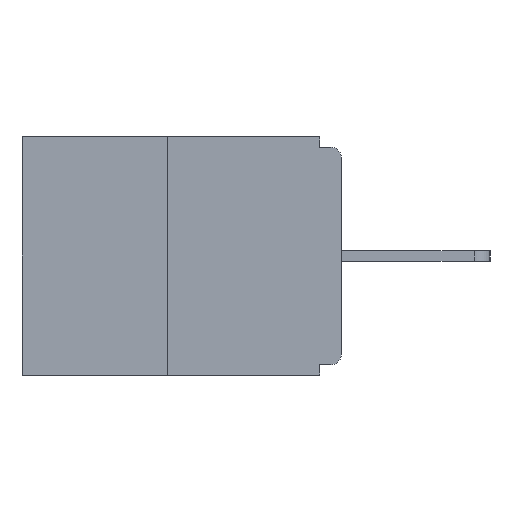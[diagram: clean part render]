
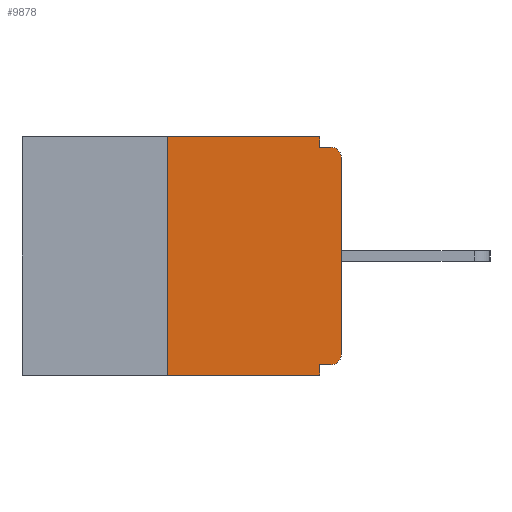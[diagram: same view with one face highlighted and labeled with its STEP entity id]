
A CAD part, left-side view. The second image highlights one B-rep face of the part: STEP entity #9878.
In plain terms, the highlighted planar face has unit normal (-1, 0, 0).
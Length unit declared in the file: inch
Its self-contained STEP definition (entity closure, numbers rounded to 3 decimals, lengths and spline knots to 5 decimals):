
#17 = CARTESIAN_POINT ( 'NONE',  ( 0., 0.25, 0. ) ) ;
#235 = DIRECTION ( 'NONE',  ( 0., 0., -1. ) ) ;
#285 = ORIENTED_EDGE ( 'NONE', *, *, #393, .F. ) ;
#359 = CARTESIAN_POINT ( 'NONE',  ( 0., 0.46, 0. ) ) ;
#393 = EDGE_CURVE ( 'NONE', #5378, #787, #4287, .T. ) ;
#433 = CARTESIAN_POINT ( 'NONE',  ( 0., 0.031, 0. ) ) ;
#787 = VERTEX_POINT ( 'NONE', #4577 ) ;
#872 = DIRECTION ( 'NONE',  ( 0., 0., -1. ) ) ;
#950 = LINE ( 'NONE', #11605, #6314 ) ;
#1039 = CARTESIAN_POINT ( 'NONE',  ( 0., 0.031, -0.015 ) ) ;
#1053 = PLANE ( 'NONE',  #10381 ) ;
#1226 = CARTESIAN_POINT ( 'NONE',  ( 0., 0.031, -0.343 ) ) ;
#1510 = VECTOR ( 'NONE', #7937, 39.37008 ) ;
#1736 = VERTEX_POINT ( 'NONE', #4170 ) ;
#2006 = VERTEX_POINT ( 'NONE', #6534 ) ;
#2143 = DIRECTION ( 'NONE',  ( 0., 0., 1. ) ) ;
#2172 = VERTEX_POINT ( 'NONE', #17 ) ;
#2188 = CARTESIAN_POINT ( 'NONE',  ( 0., 0., -0.015 ) ) ;
#2247 = VECTOR ( 'NONE', #2143, 39.37008 ) ;
#2302 = CARTESIAN_POINT ( 'NONE',  ( 0., 0.015, -0.03 ) ) ;
#2700 = AXIS2_PLACEMENT_3D ( 'NONE', #12912, #8951, #4931 ) ;
#2764 = EDGE_LOOP ( 'NONE', ( #7004, #6138, #12040, #3633, #285, #4777, #11546, #6437, #5167, #11574 ) ) ;
#2909 = CARTESIAN_POINT ( 'NONE',  ( 0., 0., 0. ) ) ;
#3272 = VECTOR ( 'NONE', #4357, 39.37008 ) ;
#3365 = EDGE_CURVE ( 'NONE', #5378, #11676, #10576, .T. ) ;
#3538 = VERTEX_POINT ( 'NONE', #1226 ) ;
#3633 = ORIENTED_EDGE ( 'NONE', *, *, #9804, .F. ) ;
#3805 = VECTOR ( 'NONE', #7777, 39.37008 ) ;
#4025 = CIRCLE ( 'NONE', #5738, 0.015 ) ;
#4141 = LINE ( 'NONE', #2188, #4601 ) ;
#4170 = CARTESIAN_POINT ( 'NONE',  ( 0., 0., -0.03 ) ) ;
#4282 = LINE ( 'NONE', #11098, #2247 ) ;
#4287 = LINE ( 'NONE', #10485, #11205 ) ;
#4319 = DIRECTION ( 'NONE',  ( -1., 0., 0. ) ) ;
#4357 = DIRECTION ( 'NONE',  ( 0., -1., 0. ) ) ;
#4483 = EDGE_CURVE ( 'NONE', #6770, #11737, #950, .T. ) ;
#4577 = CARTESIAN_POINT ( 'NONE',  ( 0., 0.031, -0.328 ) ) ;
#4599 = FACE_OUTER_BOUND ( 'NONE', #2764, .T. ) ;
#4601 = VECTOR ( 'NONE', #9280, 39.37008 ) ;
#4777 = ORIENTED_EDGE ( 'NONE', *, *, #3365, .T. ) ;
#4931 = DIRECTION ( 'NONE',  ( 0., 0., -1. ) ) ;
#5031 = CARTESIAN_POINT ( 'NONE',  ( 0., 0., -0.313 ) ) ;
#5081 = LINE ( 'NONE', #12770, #3805 ) ;
#5167 = ORIENTED_EDGE ( 'NONE', *, *, #12287, .F. ) ;
#5378 = VERTEX_POINT ( 'NONE', #8923 ) ;
#5620 = EDGE_CURVE ( 'NONE', #2172, #6770, #13023, .T. ) ;
#5738 = AXIS2_PLACEMENT_3D ( 'NONE', #2302, #4319, #235 ) ;
#6138 = ORIENTED_EDGE ( 'NONE', *, *, #12795, .F. ) ;
#6314 = VECTOR ( 'NONE', #8544, 39.37008 ) ;
#6437 = ORIENTED_EDGE ( 'NONE', *, *, #7498, .T. ) ;
#6534 = CARTESIAN_POINT ( 'NONE',  ( 0., 0.25, -0.343 ) ) ;
#6692 = VERTEX_POINT ( 'NONE', #9194 ) ;
#6770 = VERTEX_POINT ( 'NONE', #433 ) ;
#7004 = ORIENTED_EDGE ( 'NONE', *, *, #5620, .F. ) ;
#7154 = DIRECTION ( 'NONE',  ( 0., -1., 0. ) ) ;
#7236 = EDGE_CURVE ( 'NONE', #11676, #1736, #12823, .T. ) ;
#7498 = EDGE_CURVE ( 'NONE', #1736, #6692, #4025, .T. ) ;
#7777 = DIRECTION ( 'NONE',  ( 0., 0., -1. ) ) ;
#7937 = DIRECTION ( 'NONE',  ( 0., 0., 1. ) ) ;
#8115 = EDGE_CURVE ( 'NONE', #2006, #3538, #12953, .T. ) ;
#8544 = DIRECTION ( 'NONE',  ( 0., 0., -1. ) ) ;
#8923 = CARTESIAN_POINT ( 'NONE',  ( 0., 0.015, -0.328 ) ) ;
#8951 = DIRECTION ( 'NONE',  ( -1., 0., 0. ) ) ;
#8978 = CARTESIAN_POINT ( 'NONE',  ( 0., 0.46, 0. ) ) ;
#9045 = CARTESIAN_POINT ( 'NONE',  ( 0., 0.46, -0.343 ) ) ;
#9194 = CARTESIAN_POINT ( 'NONE',  ( 0., 0.015, -0.015 ) ) ;
#9280 = DIRECTION ( 'NONE',  ( 0., -1., 0. ) ) ;
#9804 = EDGE_CURVE ( 'NONE', #787, #3538, #5081, .T. ) ;
#9878 = ADVANCED_FACE ( 'NONE', ( #4599 ), #1053, .F. ) ;
#10381 = AXIS2_PLACEMENT_3D ( 'NONE', #8978, #10892, #872 ) ;
#10485 = CARTESIAN_POINT ( 'NONE',  ( 0., 0., -0.328 ) ) ;
#10576 = CIRCLE ( 'NONE', #2700, 0.015 ) ;
#10892 = DIRECTION ( 'NONE',  ( 1., 0., 0. ) ) ;
#11098 = CARTESIAN_POINT ( 'NONE',  ( 0., 0.25, 0. ) ) ;
#11205 = VECTOR ( 'NONE', #12455, 39.37008 ) ;
#11546 = ORIENTED_EDGE ( 'NONE', *, *, #7236, .T. ) ;
#11574 = ORIENTED_EDGE ( 'NONE', *, *, #4483, .F. ) ;
#11605 = CARTESIAN_POINT ( 'NONE',  ( 0., 0.031, 0. ) ) ;
#11676 = VERTEX_POINT ( 'NONE', #5031 ) ;
#11696 = VECTOR ( 'NONE', #7154, 39.37008 ) ;
#11737 = VERTEX_POINT ( 'NONE', #1039 ) ;
#12040 = ORIENTED_EDGE ( 'NONE', *, *, #8115, .T. ) ;
#12287 = EDGE_CURVE ( 'NONE', #11737, #6692, #4141, .T. ) ;
#12455 = DIRECTION ( 'NONE',  ( 0., 1., 0. ) ) ;
#12770 = CARTESIAN_POINT ( 'NONE',  ( 0., 0.031, -0.343 ) ) ;
#12795 = EDGE_CURVE ( 'NONE', #2006, #2172, #4282, .T. ) ;
#12823 = LINE ( 'NONE', #2909, #1510 ) ;
#12912 = CARTESIAN_POINT ( 'NONE',  ( 0., 0.015, -0.313 ) ) ;
#12953 = LINE ( 'NONE', #9045, #11696 ) ;
#13023 = LINE ( 'NONE', #359, #3272 ) ;
